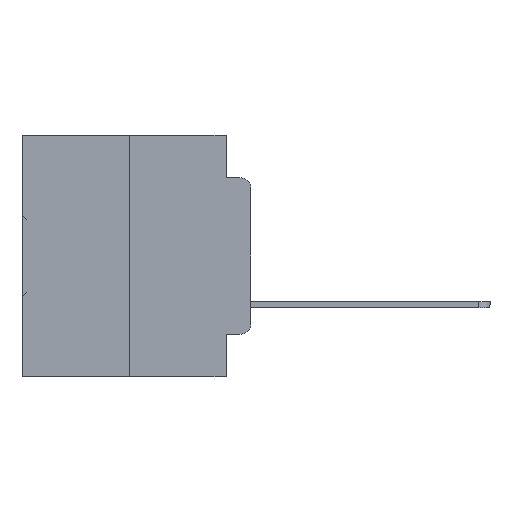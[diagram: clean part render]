
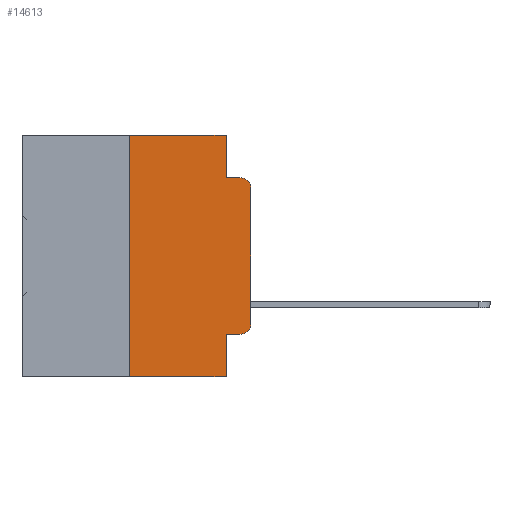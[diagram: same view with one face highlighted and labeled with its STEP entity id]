
A CAD part, left-side view. The second image highlights one B-rep face of the part: STEP entity #14613.
In plain terms, the highlighted planar face has unit normal (-1, 0, 0).
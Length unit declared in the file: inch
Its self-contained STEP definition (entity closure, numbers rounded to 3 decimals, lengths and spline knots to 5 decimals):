
#462 = CARTESIAN_POINT ( 'NONE',  ( 0., 0.473, 0. ) ) ;
#734 = DIRECTION ( 'NONE',  ( 0., 0., -1. ) ) ;
#1101 = CARTESIAN_POINT ( 'NONE',  ( 0., 0.02, -0.0885 ) ) ;
#1118 = VECTOR ( 'NONE', #7211, 39.37008 ) ;
#1419 = LINE ( 'NONE', #30219, #22790 ) ;
#1667 = CARTESIAN_POINT ( 'NONE',  ( 0., 0.051, -0.4115 ) ) ;
#1729 = DIRECTION ( 'NONE',  ( 0., 0., 1. ) ) ;
#2008 = ORIENTED_EDGE ( 'NONE', *, *, #22841, .T. ) ;
#2423 = ORIENTED_EDGE ( 'NONE', *, *, #18979, .T. ) ;
#3995 = LINE ( 'NONE', #15508, #14923 ) ;
#4273 = EDGE_CURVE ( 'NONE', #5337, #19006, #30894, .T. ) ;
#4624 = CARTESIAN_POINT ( 'NONE',  ( 0., 0.02, -0.3915 ) ) ;
#4738 = VECTOR ( 'NONE', #35555, 39.37008 ) ;
#5032 = ORIENTED_EDGE ( 'NONE', *, *, #15161, .F. ) ;
#5057 = LINE ( 'NONE', #35170, #21473 ) ;
#5337 = VERTEX_POINT ( 'NONE', #26559 ) ;
#5894 = ORIENTED_EDGE ( 'NONE', *, *, #6834, .T. ) ;
#6304 = ORIENTED_EDGE ( 'NONE', *, *, #15371, .F. ) ;
#6834 = EDGE_CURVE ( 'NONE', #5337, #30024, #1419, .T. ) ;
#7211 = DIRECTION ( 'NONE',  ( 0., -1., 0. ) ) ;
#7490 = DIRECTION ( 'NONE',  ( 0., 0., -1. ) ) ;
#7536 = ORIENTED_EDGE ( 'NONE', *, *, #16021, .T. ) ;
#9032 = CARTESIAN_POINT ( 'NONE',  ( 0., 0.02, -0.1085 ) ) ;
#9271 = EDGE_CURVE ( 'NONE', #24994, #20187, #3995, .T. ) ;
#9286 = ORIENTED_EDGE ( 'NONE', *, *, #4273, .F. ) ;
#9482 = VERTEX_POINT ( 'NONE', #1667 ) ;
#9731 = DIRECTION ( 'NONE',  ( 0., 0., 1. ) ) ;
#10137 = CIRCLE ( 'NONE', #37073, 0.02 ) ;
#11005 = DIRECTION ( 'NONE',  ( 0., 0., -1. ) ) ;
#11722 = DIRECTION ( 'NONE',  ( -1., 0., 0. ) ) ;
#13306 = DIRECTION ( 'NONE',  ( 0., -1., 0. ) ) ;
#14128 = DIRECTION ( 'NONE',  ( 1., 0., 0. ) ) ;
#14613 = ADVANCED_FACE ( 'NONE', ( #23718 ), #28887, .F. ) ;
#14788 = CARTESIAN_POINT ( 'NONE',  ( 0., 0.02, -0.4115 ) ) ;
#14923 = VECTOR ( 'NONE', #734, 39.37008 ) ;
#15161 = EDGE_CURVE ( 'NONE', #19006, #24994, #18632, .T. ) ;
#15371 = EDGE_CURVE ( 'NONE', #20187, #25748, #18552, .T. ) ;
#15508 = CARTESIAN_POINT ( 'NONE',  ( 0., 0.051, 0. ) ) ;
#16021 = EDGE_CURVE ( 'NONE', #9482, #17683, #17122, .T. ) ;
#16313 = CARTESIAN_POINT ( 'NONE',  ( 0., 0.25, 0. ) ) ;
#17122 = LINE ( 'NONE', #26140, #20114 ) ;
#17683 = VERTEX_POINT ( 'NONE', #14788 ) ;
#18311 = EDGE_LOOP ( 'NONE', ( #23047, #2423, #6304, #36850, #5032, #9286, #5894, #29776, #7536, #2008 ) ) ;
#18552 = LINE ( 'NONE', #33315, #1118 ) ;
#18632 = LINE ( 'NONE', #462, #4738 ) ;
#18979 = EDGE_CURVE ( 'NONE', #24179, #25748, #35020, .T. ) ;
#19006 = VERTEX_POINT ( 'NONE', #20158 ) ;
#20114 = VECTOR ( 'NONE', #29018, 39.37008 ) ;
#20158 = CARTESIAN_POINT ( 'NONE',  ( 0., 0.25, 0. ) ) ;
#20187 = VERTEX_POINT ( 'NONE', #30304 ) ;
#21473 = VECTOR ( 'NONE', #11005, 39.37008 ) ;
#22220 = VECTOR ( 'NONE', #1729, 39.37008 ) ;
#22790 = VECTOR ( 'NONE', #13306, 39.37008 ) ;
#22841 = EDGE_CURVE ( 'NONE', #17683, #30936, #10137, .T. ) ;
#23047 = ORIENTED_EDGE ( 'NONE', *, *, #25702, .T. ) ;
#23718 = FACE_OUTER_BOUND ( 'NONE', #18311, .T. ) ;
#24179 = VERTEX_POINT ( 'NONE', #35385 ) ;
#24329 = LINE ( 'NONE', #36019, #29235 ) ;
#24994 = VERTEX_POINT ( 'NONE', #33417 ) ;
#25702 = EDGE_CURVE ( 'NONE', #30936, #24179, #24329, .T. ) ;
#25748 = VERTEX_POINT ( 'NONE', #1101 ) ;
#26140 = CARTESIAN_POINT ( 'NONE',  ( 0., 0.051, -0.4115 ) ) ;
#26456 = AXIS2_PLACEMENT_3D ( 'NONE', #9032, #11722, #37811 ) ;
#26559 = CARTESIAN_POINT ( 'NONE',  ( 0., 0.25, -0.5 ) ) ;
#28887 = PLANE ( 'NONE',  #37792 ) ;
#29018 = DIRECTION ( 'NONE',  ( 0., -1., 0. ) ) ;
#29235 = VECTOR ( 'NONE', #9731, 39.37008 ) ;
#29480 = EDGE_CURVE ( 'NONE', #9482, #30024, #5057, .T. ) ;
#29682 = CARTESIAN_POINT ( 'NONE',  ( 0., 0., -0.3915 ) ) ;
#29776 = ORIENTED_EDGE ( 'NONE', *, *, #29480, .F. ) ;
#30024 = VERTEX_POINT ( 'NONE', #35125 ) ;
#30219 = CARTESIAN_POINT ( 'NONE',  ( 0., 0.473, -0.5 ) ) ;
#30304 = CARTESIAN_POINT ( 'NONE',  ( 0., 0.051, -0.0885 ) ) ;
#30894 = LINE ( 'NONE', #16313, #22220 ) ;
#30936 = VERTEX_POINT ( 'NONE', #29682 ) ;
#33315 = CARTESIAN_POINT ( 'NONE',  ( 0., 0.051, -0.0885 ) ) ;
#33417 = CARTESIAN_POINT ( 'NONE',  ( 0., 0.051, 0. ) ) ;
#33778 = DIRECTION ( 'NONE',  ( -1., 0., 0. ) ) ;
#34638 = DIRECTION ( 'NONE',  ( 0., 0., -1. ) ) ;
#35020 = CIRCLE ( 'NONE', #26456, 0.02 ) ;
#35125 = CARTESIAN_POINT ( 'NONE',  ( 0., 0.051, -0.5 ) ) ;
#35170 = CARTESIAN_POINT ( 'NONE',  ( 0., 0.051, 0. ) ) ;
#35385 = CARTESIAN_POINT ( 'NONE',  ( 0., 0., -0.1085 ) ) ;
#35408 = CARTESIAN_POINT ( 'NONE',  ( 0., 0.473, 0. ) ) ;
#35555 = DIRECTION ( 'NONE',  ( 0., -1., 0. ) ) ;
#36019 = CARTESIAN_POINT ( 'NONE',  ( 0., 0., 0. ) ) ;
#36850 = ORIENTED_EDGE ( 'NONE', *, *, #9271, .F. ) ;
#37073 = AXIS2_PLACEMENT_3D ( 'NONE', #4624, #33778, #7490 ) ;
#37792 = AXIS2_PLACEMENT_3D ( 'NONE', #35408, #14128, #34638 ) ;
#37811 = DIRECTION ( 'NONE',  ( 0., 0., -1. ) ) ;
